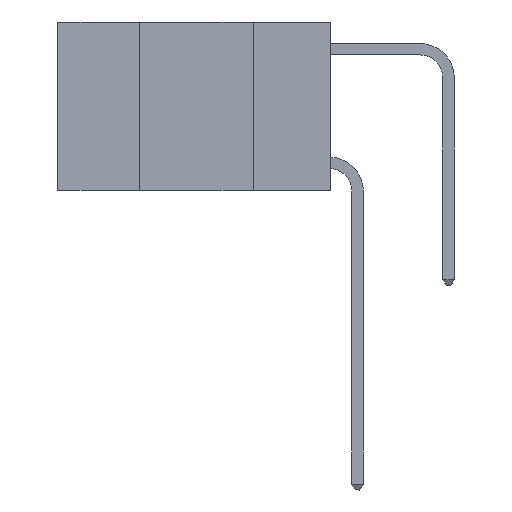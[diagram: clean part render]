
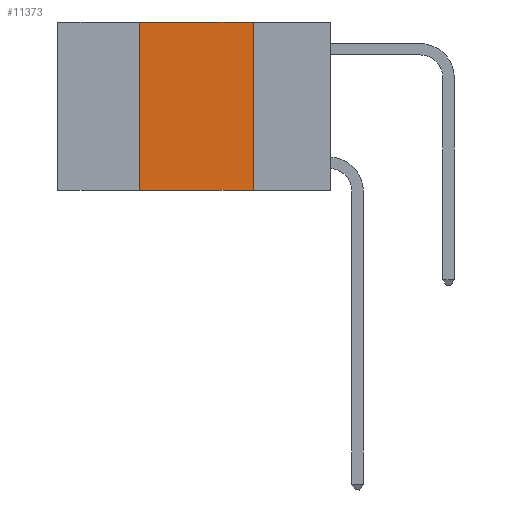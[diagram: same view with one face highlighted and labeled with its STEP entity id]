
A CAD part, left-side view. The second image highlights one B-rep face of the part: STEP entity #11373.
In plain terms, the highlighted planar face has unit normal (-1, 0, 0).
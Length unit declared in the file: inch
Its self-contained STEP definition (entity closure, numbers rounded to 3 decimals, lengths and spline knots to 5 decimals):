
#906 = LINE ( 'NONE', #4724, #14396 ) ;
#1009 = DIRECTION ( 'NONE',  ( 0., -1., 0. ) ) ;
#1681 = EDGE_CURVE ( 'NONE', #7586, #16967, #16313, .T. ) ;
#2075 = DIRECTION ( 'NONE',  ( 0., 0., -1. ) ) ;
#2203 = EDGE_CURVE ( 'NONE', #16967, #14487, #4435, .T. ) ;
#2211 = EDGE_CURVE ( 'NONE', #15580, #7586, #906, .T. ) ;
#2232 = EDGE_CURVE ( 'NONE', #15580, #14487, #17946, .T. ) ;
#2786 = DIRECTION ( 'NONE',  ( 0., 0., 1. ) ) ;
#2875 = CARTESIAN_POINT ( 'NONE',  ( 0., 0.17, 0. ) ) ;
#3619 = CARTESIAN_POINT ( 'NONE',  ( 0., 0.42, -0.37 ) ) ;
#4435 = LINE ( 'NONE', #2875, #11319 ) ;
#4724 = CARTESIAN_POINT ( 'NONE',  ( 0., 0.42, 0. ) ) ;
#5057 = CARTESIAN_POINT ( 'NONE',  ( 0., 0.6, 0. ) ) ;
#5118 = DIRECTION ( 'NONE',  ( 0., 0., -1. ) ) ;
#5139 = FACE_OUTER_BOUND ( 'NONE', #11791, .T. ) ;
#5443 = DIRECTION ( 'NONE',  ( 0., -1., 0. ) ) ;
#6694 = AXIS2_PLACEMENT_3D ( 'NONE', #5057, #13211, #5118 ) ;
#7023 = CARTESIAN_POINT ( 'NONE',  ( 0., 0.17, -0.37 ) ) ;
#7586 = VERTEX_POINT ( 'NONE', #7738 ) ;
#7738 = CARTESIAN_POINT ( 'NONE',  ( 0., 0.42, 0. ) ) ;
#10322 = ORIENTED_EDGE ( 'NONE', *, *, #2211, .F. ) ;
#10552 = PLANE ( 'NONE',  #6694 ) ;
#10555 = CARTESIAN_POINT ( 'NONE',  ( 0., 0.17, 0. ) ) ;
#11319 = VECTOR ( 'NONE', #2075, 39.37008 ) ;
#11373 = ADVANCED_FACE ( 'NONE', ( #5139 ), #10552, .F. ) ;
#11791 = EDGE_LOOP ( 'NONE', ( #16568, #13429, #10322, #17376 ) ) ;
#12344 = CARTESIAN_POINT ( 'NONE',  ( 0., 0.6, 0. ) ) ;
#13211 = DIRECTION ( 'NONE',  ( 1., 0., 0. ) ) ;
#13429 = ORIENTED_EDGE ( 'NONE', *, *, #1681, .F. ) ;
#13977 = VECTOR ( 'NONE', #1009, 39.37008 ) ;
#14396 = VECTOR ( 'NONE', #2786, 39.37008 ) ;
#14487 = VERTEX_POINT ( 'NONE', #7023 ) ;
#15365 = CARTESIAN_POINT ( 'NONE',  ( 0., 0.6, -0.37 ) ) ;
#15580 = VERTEX_POINT ( 'NONE', #3619 ) ;
#16313 = LINE ( 'NONE', #12344, #17122 ) ;
#16568 = ORIENTED_EDGE ( 'NONE', *, *, #2203, .F. ) ;
#16967 = VERTEX_POINT ( 'NONE', #10555 ) ;
#17122 = VECTOR ( 'NONE', #5443, 39.37008 ) ;
#17376 = ORIENTED_EDGE ( 'NONE', *, *, #2232, .T. ) ;
#17946 = LINE ( 'NONE', #15365, #13977 ) ;
